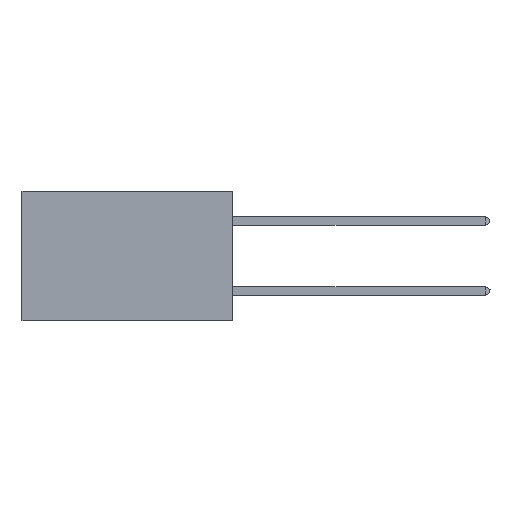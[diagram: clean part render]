
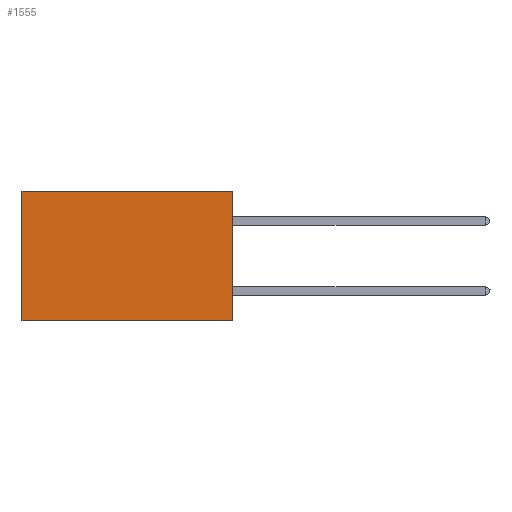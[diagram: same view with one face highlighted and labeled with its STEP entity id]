
A CAD part, left-side view. The second image highlights one B-rep face of the part: STEP entity #1555.
In plain terms, the highlighted planar face has unit normal (-1, 0, 0).
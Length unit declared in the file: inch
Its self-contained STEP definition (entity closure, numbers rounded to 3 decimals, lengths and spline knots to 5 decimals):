
#260 = DIRECTION ( 'NONE',  ( 1., 0., 0. ) ) ;
#504 = LINE ( 'NONE', #2928, #11056 ) ;
#1511 = FACE_OUTER_BOUND ( 'NONE', #24306, .T. ) ;
#1555 = ADVANCED_FACE ( 'NONE', ( #1511 ), #24373, .F. ) ;
#2080 = LINE ( 'NONE', #22083, #24963 ) ;
#2614 = EDGE_CURVE ( 'NONE', #4379, #6587, #18340, .T. ) ;
#2928 = CARTESIAN_POINT ( 'NONE',  ( 0.2875, 0., -0.37 ) ) ;
#3161 = ORIENTED_EDGE ( 'NONE', *, *, #2614, .F. ) ;
#4379 = VERTEX_POINT ( 'NONE', #11905 ) ;
#5292 = VERTEX_POINT ( 'NONE', #18805 ) ;
#6471 = ORIENTED_EDGE ( 'NONE', *, *, #25579, .T. ) ;
#6587 = VERTEX_POINT ( 'NONE', #21006 ) ;
#8368 = CARTESIAN_POINT ( 'NONE',  ( 0.2875, 0.6, 0. ) ) ;
#11056 = VECTOR ( 'NONE', #17098, 39.37008 ) ;
#11905 = CARTESIAN_POINT ( 'NONE',  ( 0.2875, 0., 0. ) ) ;
#12129 = DIRECTION ( 'NONE',  ( 0., 0., -1. ) ) ;
#13016 = VECTOR ( 'NONE', #19340, 39.37008 ) ;
#14051 = DIRECTION ( 'NONE',  ( 0., 1., 0. ) ) ;
#14553 = VERTEX_POINT ( 'NONE', #8368 ) ;
#15332 = CARTESIAN_POINT ( 'NONE',  ( 0.2875, 0., 0. ) ) ;
#17098 = DIRECTION ( 'NONE',  ( 0., 1., 0. ) ) ;
#17127 = EDGE_CURVE ( 'NONE', #14553, #5292, #2080, .T. ) ;
#17708 = ORIENTED_EDGE ( 'NONE', *, *, #17900, .F. ) ;
#17900 = EDGE_CURVE ( 'NONE', #6587, #5292, #504, .T. ) ;
#17956 = ORIENTED_EDGE ( 'NONE', *, *, #17127, .T. ) ;
#18340 = LINE ( 'NONE', #15332, #13016 ) ;
#18366 = DIRECTION ( 'NONE',  ( 0., 0., -1. ) ) ;
#18805 = CARTESIAN_POINT ( 'NONE',  ( 0.2875, 0.6, -0.37 ) ) ;
#19340 = DIRECTION ( 'NONE',  ( 0., 0., -1. ) ) ;
#21006 = CARTESIAN_POINT ( 'NONE',  ( 0.2875, 0., -0.37 ) ) ;
#21028 = LINE ( 'NONE', #22460, #24535 ) ;
#22083 = CARTESIAN_POINT ( 'NONE',  ( 0.2875, 0.6, 0. ) ) ;
#22460 = CARTESIAN_POINT ( 'NONE',  ( 0.2875, 0., 0. ) ) ;
#24197 = CARTESIAN_POINT ( 'NONE',  ( 0.2875, 0., 0. ) ) ;
#24306 = EDGE_LOOP ( 'NONE', ( #17956, #17708, #3161, #6471 ) ) ;
#24373 = PLANE ( 'NONE',  #24380 ) ;
#24380 = AXIS2_PLACEMENT_3D ( 'NONE', #24197, #260, #12129 ) ;
#24535 = VECTOR ( 'NONE', #14051, 39.37008 ) ;
#24963 = VECTOR ( 'NONE', #18366, 39.37008 ) ;
#25579 = EDGE_CURVE ( 'NONE', #4379, #14553, #21028, .T. ) ;
